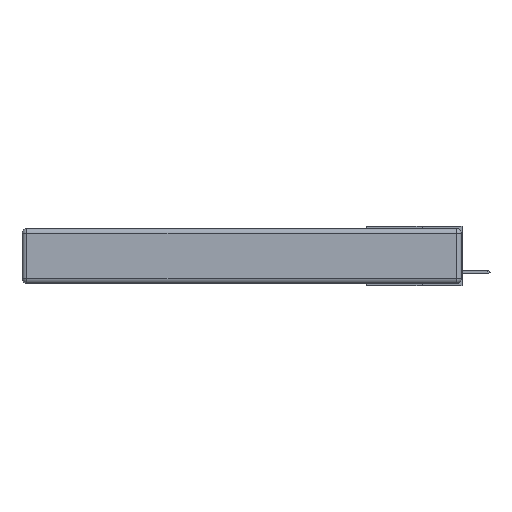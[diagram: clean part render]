
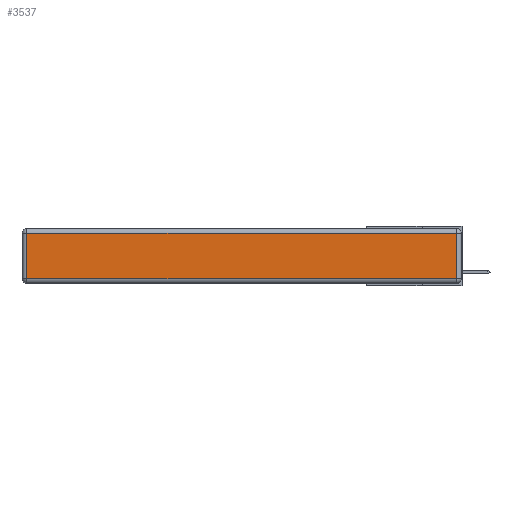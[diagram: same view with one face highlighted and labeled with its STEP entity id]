
A CAD part, left-side view. The second image highlights one B-rep face of the part: STEP entity #3537.
In plain terms, the highlighted planar face has unit normal (-1, 0, 0).
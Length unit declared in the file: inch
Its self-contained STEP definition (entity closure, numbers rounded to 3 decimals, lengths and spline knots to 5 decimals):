
#526 = VECTOR ( 'NONE', #6908, 39.37008 ) ;
#898 = ORIENTED_EDGE ( 'NONE', *, *, #5693, .T. ) ;
#1524 = DIRECTION ( 'NONE',  ( 0., 0., 1. ) ) ;
#1773 = AXIS2_PLACEMENT_3D ( 'NONE', #2243, #7950, #1524 ) ;
#1985 = ORIENTED_EDGE ( 'NONE', *, *, #2896, .T. ) ;
#2236 = VECTOR ( 'NONE', #9562, 39.37008 ) ;
#2243 = CARTESIAN_POINT ( 'NONE',  ( 0., 0., -0.343 ) ) ;
#2827 = LINE ( 'NONE', #2965, #2236 ) ;
#2896 = EDGE_CURVE ( 'NONE', #6917, #4267, #11518, .T. ) ;
#2965 = CARTESIAN_POINT ( 'NONE',  ( 0., 2.75, -0.03 ) ) ;
#3430 = LINE ( 'NONE', #4175, #526 ) ;
#3537 = ADVANCED_FACE ( 'NONE', ( #4910 ), #11578, .T. ) ;
#3619 = CARTESIAN_POINT ( 'NONE',  ( 0., 0.03, -0.313 ) ) ;
#4160 = VERTEX_POINT ( 'NONE', #4251 ) ;
#4175 = CARTESIAN_POINT ( 'NONE',  ( 0., 2.72, -0.343 ) ) ;
#4251 = CARTESIAN_POINT ( 'NONE',  ( 0., 2.72, -0.03 ) ) ;
#4267 = VERTEX_POINT ( 'NONE', #3619 ) ;
#4718 = LINE ( 'NONE', #7904, #6574 ) ;
#4910 = FACE_OUTER_BOUND ( 'NONE', #8565, .T. ) ;
#5693 = EDGE_CURVE ( 'NONE', #9343, #4160, #2827, .T. ) ;
#6176 = DIRECTION ( 'NONE',  ( 0., -1., 0. ) ) ;
#6574 = VECTOR ( 'NONE', #7864, 39.37008 ) ;
#6726 = CARTESIAN_POINT ( 'NONE',  ( 0., 2.72, -0.313 ) ) ;
#6908 = DIRECTION ( 'NONE',  ( 0., 0., -1. ) ) ;
#6917 = VERTEX_POINT ( 'NONE', #6726 ) ;
#7864 = DIRECTION ( 'NONE',  ( 0., 0., 1. ) ) ;
#7904 = CARTESIAN_POINT ( 'NONE',  ( 0., 0.03, -0.343 ) ) ;
#7950 = DIRECTION ( 'NONE',  ( -1., 0., 0. ) ) ;
#8565 = EDGE_LOOP ( 'NONE', ( #1985, #10495, #898, #10323 ) ) ;
#8894 = CARTESIAN_POINT ( 'NONE',  ( 0., 0., -0.313 ) ) ;
#9343 = VERTEX_POINT ( 'NONE', #11954 ) ;
#9481 = VECTOR ( 'NONE', #6176, 39.37008 ) ;
#9562 = DIRECTION ( 'NONE',  ( 0., 1., 0. ) ) ;
#9718 = EDGE_CURVE ( 'NONE', #4267, #9343, #4718, .T. ) ;
#10181 = EDGE_CURVE ( 'NONE', #4160, #6917, #3430, .T. ) ;
#10323 = ORIENTED_EDGE ( 'NONE', *, *, #10181, .T. ) ;
#10495 = ORIENTED_EDGE ( 'NONE', *, *, #9718, .T. ) ;
#11518 = LINE ( 'NONE', #8894, #9481 ) ;
#11578 = PLANE ( 'NONE',  #1773 ) ;
#11954 = CARTESIAN_POINT ( 'NONE',  ( 0., 0.03, -0.03 ) ) ;
